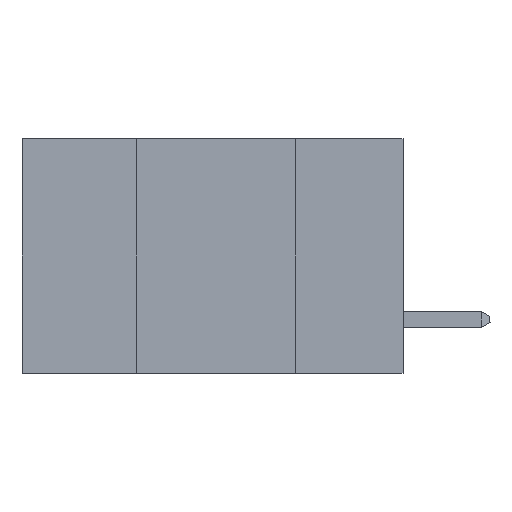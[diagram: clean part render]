
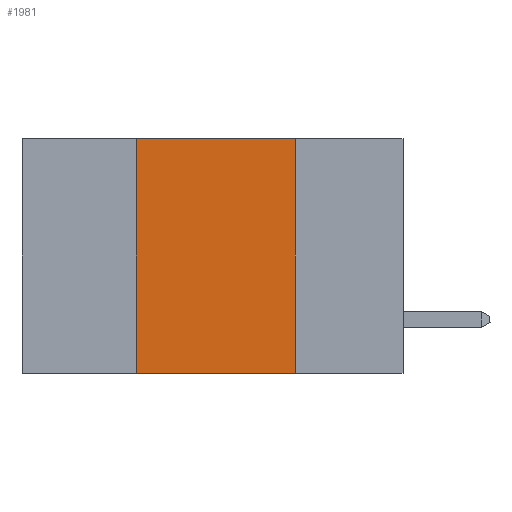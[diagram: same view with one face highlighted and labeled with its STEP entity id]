
A CAD part, left-side view. The second image highlights one B-rep face of the part: STEP entity #1981.
In plain terms, the highlighted planar face has unit normal (-1, 0, 0).
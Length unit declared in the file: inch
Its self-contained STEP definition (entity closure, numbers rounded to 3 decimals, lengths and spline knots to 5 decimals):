
#277 = ORIENTED_EDGE ( 'NONE', *, *, #17071, .F. ) ;
#422 = LINE ( 'NONE', #11621, #2778 ) ;
#614 = CARTESIAN_POINT ( 'NONE',  ( 0., 0.42, 0. ) ) ;
#1313 = DIRECTION ( 'NONE',  ( 0., -1., 0. ) ) ;
#1981 = ADVANCED_FACE ( 'NONE', ( #13944 ), #4124, .F. ) ;
#2393 = VECTOR ( 'NONE', #9593, 39.37008 ) ;
#2778 = VECTOR ( 'NONE', #1313, 39.37008 ) ;
#3025 = CARTESIAN_POINT ( 'NONE',  ( 0., 0.17, -0.37 ) ) ;
#3395 = ORIENTED_EDGE ( 'NONE', *, *, #3585, .F. ) ;
#3585 = EDGE_CURVE ( 'NONE', #11754, #8751, #10698, .T. ) ;
#4124 = PLANE ( 'NONE',  #11710 ) ;
#6725 = DIRECTION ( 'NONE',  ( 1., 0., 0. ) ) ;
#6842 = LINE ( 'NONE', #10884, #2393 ) ;
#7096 = VECTOR ( 'NONE', #11558, 39.37008 ) ;
#8751 = VERTEX_POINT ( 'NONE', #13995 ) ;
#9552 = ORIENTED_EDGE ( 'NONE', *, *, #10794, .F. ) ;
#9593 = DIRECTION ( 'NONE',  ( 0., -1., 0. ) ) ;
#10698 = LINE ( 'NONE', #614, #7096 ) ;
#10794 = EDGE_CURVE ( 'NONE', #13181, #16926, #15570, .T. ) ;
#10884 = CARTESIAN_POINT ( 'NONE',  ( 0., 0.6, -0.37 ) ) ;
#11386 = EDGE_LOOP ( 'NONE', ( #9552, #277, #3395, #12552 ) ) ;
#11558 = DIRECTION ( 'NONE',  ( 0., 0., 1. ) ) ;
#11621 = CARTESIAN_POINT ( 'NONE',  ( 0., 0.6, 0. ) ) ;
#11710 = AXIS2_PLACEMENT_3D ( 'NONE', #13612, #6725, #13435 ) ;
#11754 = VERTEX_POINT ( 'NONE', #15524 ) ;
#11969 = VECTOR ( 'NONE', #13886, 39.37008 ) ;
#12500 = EDGE_CURVE ( 'NONE', #11754, #16926, #6842, .T. ) ;
#12552 = ORIENTED_EDGE ( 'NONE', *, *, #12500, .T. ) ;
#13181 = VERTEX_POINT ( 'NONE', #15606 ) ;
#13435 = DIRECTION ( 'NONE',  ( 0., 0., -1. ) ) ;
#13612 = CARTESIAN_POINT ( 'NONE',  ( 0., 0.6, 0. ) ) ;
#13886 = DIRECTION ( 'NONE',  ( 0., 0., -1. ) ) ;
#13944 = FACE_OUTER_BOUND ( 'NONE', #11386, .T. ) ;
#13995 = CARTESIAN_POINT ( 'NONE',  ( 0., 0.42, 0. ) ) ;
#15524 = CARTESIAN_POINT ( 'NONE',  ( 0., 0.42, -0.37 ) ) ;
#15570 = LINE ( 'NONE', #16766, #11969 ) ;
#15606 = CARTESIAN_POINT ( 'NONE',  ( 0., 0.17, 0. ) ) ;
#16766 = CARTESIAN_POINT ( 'NONE',  ( 0., 0.17, 0. ) ) ;
#16926 = VERTEX_POINT ( 'NONE', #3025 ) ;
#17071 = EDGE_CURVE ( 'NONE', #8751, #13181, #422, .T. ) ;
